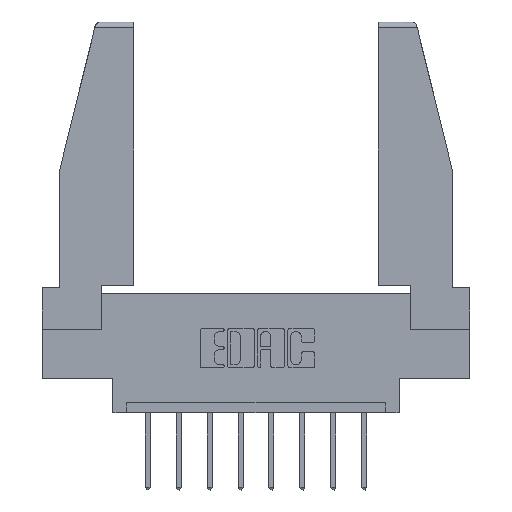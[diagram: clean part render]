
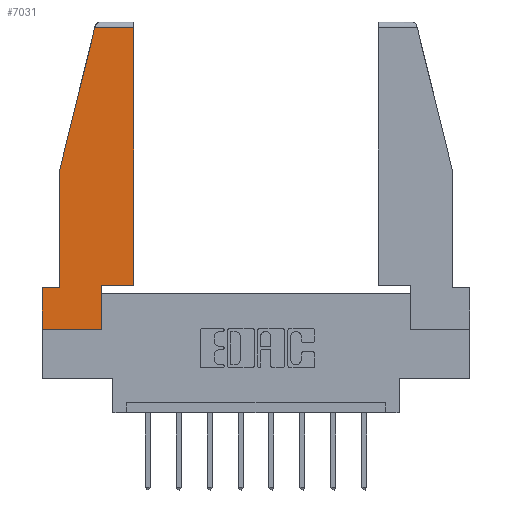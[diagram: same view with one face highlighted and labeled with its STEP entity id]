
A CAD part, top view. The second image highlights one B-rep face of the part: STEP entity #7031.
In plain terms, the highlighted planar face has unit normal (0, 0, 1).
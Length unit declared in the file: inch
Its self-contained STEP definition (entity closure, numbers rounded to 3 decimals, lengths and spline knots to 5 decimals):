
#170 = CARTESIAN_POINT ( 'NONE',  ( 0.271, 1.55, 0. ) ) ;
#582 = LINE ( 'NONE', #10865, #6820 ) ;
#709 = CARTESIAN_POINT ( 'NONE',  ( 0.461, 0.223, 0. ) ) ;
#722 = ORIENTED_EDGE ( 'NONE', *, *, #8678, .T. ) ;
#752 = VECTOR ( 'NONE', #3197, 39.37008 ) ;
#937 = VECTOR ( 'NONE', #5292, 39.37008 ) ;
#1058 = LINE ( 'NONE', #11057, #9958 ) ;
#1059 = VERTEX_POINT ( 'NONE', #3263 ) ;
#1166 = LINE ( 'NONE', #2679, #8528 ) ;
#1544 = ORIENTED_EDGE ( 'NONE', *, *, #3492, .T. ) ;
#1875 = CARTESIAN_POINT ( 'NONE',  ( 0., 0.21, 0. ) ) ;
#2335 = CARTESIAN_POINT ( 'NONE',  ( 0., 0., 0. ) ) ;
#2438 = CARTESIAN_POINT ( 'NONE',  ( 0.297, 0., 0. ) ) ;
#2501 = DIRECTION ( 'NONE',  ( 1., 0., 0. ) ) ;
#2679 = CARTESIAN_POINT ( 'NONE',  ( 0.461, 0.223, 0. ) ) ;
#3197 = DIRECTION ( 'NONE',  ( -0.239, -0.971, 0. ) ) ;
#3263 = CARTESIAN_POINT ( 'NONE',  ( 0.086, 0.21, 0. ) ) ;
#3387 = EDGE_CURVE ( 'NONE', #8997, #12404, #11582, .T. ) ;
#3464 = ORIENTED_EDGE ( 'NONE', *, *, #12387, .T. ) ;
#3492 = EDGE_CURVE ( 'NONE', #11211, #10461, #11723, .T. ) ;
#3710 = ORIENTED_EDGE ( 'NONE', *, *, #5213, .T. ) ;
#3899 = VECTOR ( 'NONE', #8475, 39.37008 ) ;
#3973 = VECTOR ( 'NONE', #10982, 39.37008 ) ;
#4400 = CARTESIAN_POINT ( 'NONE',  ( 0., 1.52, 0. ) ) ;
#4843 = CARTESIAN_POINT ( 'NONE',  ( 0.2636, 1.52, 0. ) ) ;
#4975 = LINE ( 'NONE', #6750, #6050 ) ;
#5213 = EDGE_CURVE ( 'NONE', #9184, #10157, #1058, .T. ) ;
#5292 = DIRECTION ( 'NONE',  ( -1., 0., 0. ) ) ;
#5805 = EDGE_LOOP ( 'NONE', ( #9628, #9887, #11690, #722, #3464, #9085, #1544, #8363, #3710 ) ) ;
#6050 = VECTOR ( 'NONE', #11774, 39.37008 ) ;
#6580 = EDGE_CURVE ( 'NONE', #10157, #8997, #1166, .T. ) ;
#6750 = CARTESIAN_POINT ( 'NONE',  ( 0., 0.21, 0. ) ) ;
#6820 = VECTOR ( 'NONE', #7768, 39.37008 ) ;
#6908 = VERTEX_POINT ( 'NONE', #12871 ) ;
#7031 = ADVANCED_FACE ( 'NONE', ( #7749 ), #10230, .T. ) ;
#7749 = FACE_OUTER_BOUND ( 'NONE', #5805, .T. ) ;
#7768 = DIRECTION ( 'NONE',  ( -1., 0., 0. ) ) ;
#7803 = AXIS2_PLACEMENT_3D ( 'NONE', #10064, #8179, #12038 ) ;
#7959 = CARTESIAN_POINT ( 'NONE',  ( 0.297, 0., 0. ) ) ;
#8102 = LINE ( 'NONE', #2438, #3899 ) ;
#8179 = DIRECTION ( 'NONE',  ( 0., 0., 1. ) ) ;
#8363 = ORIENTED_EDGE ( 'NONE', *, *, #10741, .T. ) ;
#8475 = DIRECTION ( 'NONE',  ( 0., 1., 0. ) ) ;
#8497 = CARTESIAN_POINT ( 'NONE',  ( 0., 0., 0. ) ) ;
#8528 = VECTOR ( 'NONE', #10719, 39.37008 ) ;
#8678 = EDGE_CURVE ( 'NONE', #6908, #1059, #9255, .T. ) ;
#8997 = VERTEX_POINT ( 'NONE', #10727 ) ;
#9085 = ORIENTED_EDGE ( 'NONE', *, *, #11504, .T. ) ;
#9184 = VERTEX_POINT ( 'NONE', #12385 ) ;
#9255 = LINE ( 'NONE', #9951, #3973 ) ;
#9628 = ORIENTED_EDGE ( 'NONE', *, *, #6580, .T. ) ;
#9887 = ORIENTED_EDGE ( 'NONE', *, *, #3387, .T. ) ;
#9951 = CARTESIAN_POINT ( 'NONE',  ( 0.086, 0.8, 0. ) ) ;
#9958 = VECTOR ( 'NONE', #10285, 39.37008 ) ;
#10064 = CARTESIAN_POINT ( 'NONE',  ( 0., 0., 0. ) ) ;
#10157 = VERTEX_POINT ( 'NONE', #709 ) ;
#10230 = PLANE ( 'NONE',  #7803 ) ;
#10241 = VERTEX_POINT ( 'NONE', #1875 ) ;
#10285 = DIRECTION ( 'NONE',  ( 1., 0., 0. ) ) ;
#10461 = VERTEX_POINT ( 'NONE', #7959 ) ;
#10640 = EDGE_CURVE ( 'NONE', #12404, #6908, #11706, .T. ) ;
#10719 = DIRECTION ( 'NONE',  ( 0., 1., 0. ) ) ;
#10727 = CARTESIAN_POINT ( 'NONE',  ( 0.461, 1.52, 0. ) ) ;
#10741 = EDGE_CURVE ( 'NONE', #10461, #9184, #8102, .T. ) ;
#10865 = CARTESIAN_POINT ( 'NONE',  ( 0., 0.21, 0. ) ) ;
#10982 = DIRECTION ( 'NONE',  ( 0., -1., 0. ) ) ;
#11057 = CARTESIAN_POINT ( 'NONE',  ( 0.297, 0.223, 0. ) ) ;
#11108 = VECTOR ( 'NONE', #2501, 39.37008 ) ;
#11211 = VERTEX_POINT ( 'NONE', #2335 ) ;
#11504 = EDGE_CURVE ( 'NONE', #10241, #11211, #4975, .T. ) ;
#11582 = LINE ( 'NONE', #4400, #937 ) ;
#11690 = ORIENTED_EDGE ( 'NONE', *, *, #10640, .T. ) ;
#11706 = LINE ( 'NONE', #170, #752 ) ;
#11723 = LINE ( 'NONE', #8497, #11108 ) ;
#11774 = DIRECTION ( 'NONE',  ( 0., -1., 0. ) ) ;
#12038 = DIRECTION ( 'NONE',  ( 1., 0., 0. ) ) ;
#12385 = CARTESIAN_POINT ( 'NONE',  ( 0.297, 0.223, 0. ) ) ;
#12387 = EDGE_CURVE ( 'NONE', #1059, #10241, #582, .T. ) ;
#12404 = VERTEX_POINT ( 'NONE', #4843 ) ;
#12871 = CARTESIAN_POINT ( 'NONE',  ( 0.086, 0.8, 0. ) ) ;
